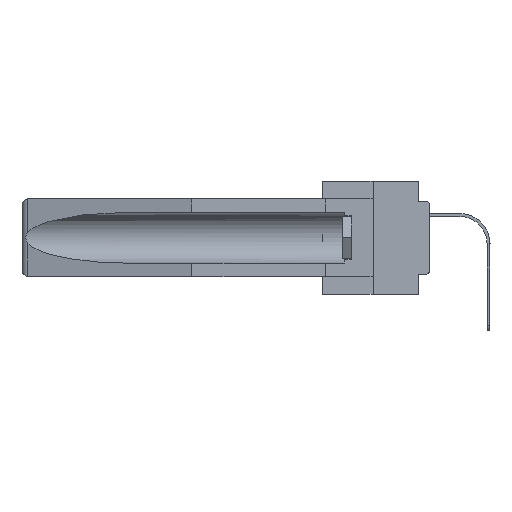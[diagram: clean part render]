
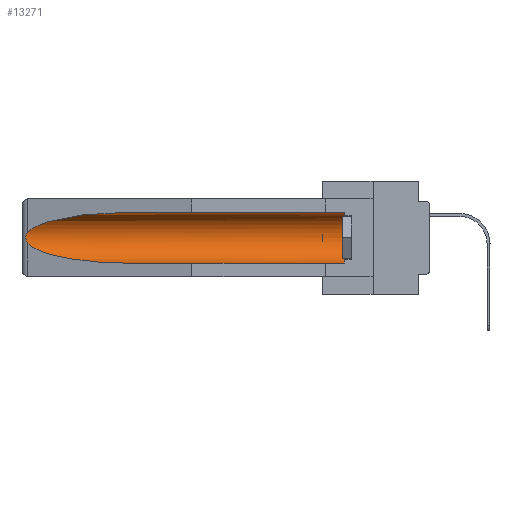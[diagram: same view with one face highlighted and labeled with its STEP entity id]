
A CAD part, left-side view. The second image highlights one B-rep face of the part: STEP entity #13271.
In plain terms, the highlighted cylindrical face has radius 2.857 mm (diameter 5.715 mm), a partial arc.
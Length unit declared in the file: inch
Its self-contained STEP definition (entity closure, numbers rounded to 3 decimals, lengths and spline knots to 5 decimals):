
#150 = CARTESIAN_POINT ( 'NONE',  ( 0.25451, 1.48313, -0.24835 ) ) ;
#886 = CARTESIAN_POINT ( 'NONE',  ( 0.155, -0.30754, -0.1715 ) ) ;
#1097 = CYLINDRICAL_SURFACE ( 'NONE', #25781, 0.1125 ) ;
#1525 =( BOUNDED_CURVE ( )  B_SPLINE_CURVE ( 3, ( #13290, #150, #25450, #12504 ),
 .UNSPECIFIED., .F., .F. ) 
 B_SPLINE_CURVE_WITH_KNOTS ( ( 4, 4 ),
 ( 0.1948, 1.5708 ),
 .UNSPECIFIED. ) 
 CURVE ( )  GEOMETRIC_REPRESENTATION_ITEM ( )  RATIONAL_B_SPLINE_CURVE ( ( 1., 0.848, 0.848, 1. ) ) 
 REPRESENTATION_ITEM ( '' )  );
#1773 = ORIENTED_EDGE ( 'NONE', *, *, #26833, .T. ) ;
#2119 = CARTESIAN_POINT ( 'NONE',  ( 0.26597, 1.5296, -0.19026 ) ) ;
#2319 = CARTESIAN_POINT ( 'NONE',  ( 0.2675, 1.53308, -0.16763 ) ) ;
#3517 = CARTESIAN_POINT ( 'NONE',  ( 0.26537, 1.52718, -0.19328 ) ) ;
#3877 = VERTEX_POINT ( 'NONE', #23800 ) ;
#5103 = DIRECTION ( 'NONE',  ( 0., 1., 0. ) ) ;
#5175 = CARTESIAN_POINT ( 'NONE',  ( 0.2673, 1.5327, -0.16383 ) ) ;
#5711 = ORIENTED_EDGE ( 'NONE', *, *, #33424, .T. ) ;
#6101 = VECTOR ( 'NONE', #5103, 39.37008 ) ;
#7322 = CARTESIAN_POINT ( 'NONE',  ( 0.155, 1.07973, -0.059 ) ) ;
#7371 = DIRECTION ( 'NONE',  ( 0., 1., 0. ) ) ;
#7547 = VERTEX_POINT ( 'NONE', #15818 ) ;
#7668 = CARTESIAN_POINT ( 'NONE',  ( 0.155, 0.126, -0.1715 ) ) ;
#8197 = CARTESIAN_POINT ( 'NONE',  ( 0.26537, 1.52718, -0.14972 ) ) ;
#8432 = DIRECTION ( 'NONE',  ( 0., 1., 0. ) ) ;
#8518 = LINE ( 'NONE', #27559, #6101 ) ;
#9685 = VERTEX_POINT ( 'NONE', #21277 ) ;
#9773 = EDGE_LOOP ( 'NONE', ( #1773, #10721, #37394, #25872, #37414, #5711 ) ) ;
#10721 = ORIENTED_EDGE ( 'NONE', *, *, #16939, .T. ) ;
#11472 = CARTESIAN_POINT ( 'NONE',  ( 0.155, -0.30754, -0.059 ) ) ;
#12179 = AXIS2_PLACEMENT_3D ( 'NONE', #7668, #26083, #20226 ) ;
#12504 = CARTESIAN_POINT ( 'NONE',  ( 0.155, 1.07973, -0.284 ) ) ;
#13271 = ADVANCED_FACE ( 'NONE', ( #28650 ), #1097, .F. ) ;
#13290 = CARTESIAN_POINT ( 'NONE',  ( 0.26537, 1.52718, -0.19328 ) ) ;
#13549 = CARTESIAN_POINT ( 'NONE',  ( 0.155, 0.126, -0.059 ) ) ;
#13828 = DIRECTION ( 'NONE',  ( 0., 0., 1. ) ) ;
#15818 = CARTESIAN_POINT ( 'NONE',  ( 0.155, 1.07973, -0.284 ) ) ;
#16831 = B_SPLINE_CURVE_WITH_KNOTS ( 'NONE', 3,
 ( #8197, #20567, #30084, #5175, #2319, #27030, #17516, #29884, #2119, #3517 ),
 .UNSPECIFIED., .F., .F.,
 ( 4, 2, 2, 2, 4 ),
 ( 0., 0.00029, 0.00058, 0.00087, 0.00117 ),
 .UNSPECIFIED. ) ;
#16939 = EDGE_CURVE ( 'NONE', #3877, #18873, #16831, .T. ) ;
#17449 = VERTEX_POINT ( 'NONE', #13549 ) ;
#17516 = CARTESIAN_POINT ( 'NONE',  ( 0.2673, 1.53269, -0.17917 ) ) ;
#17677 = EDGE_CURVE ( 'NONE', #18873, #7547, #1525, .T. ) ;
#18806 = VECTOR ( 'NONE', #8432, 39.37008 ) ;
#18873 = VERTEX_POINT ( 'NONE', #26953 ) ;
#19395 =( BOUNDED_CURVE ( )  B_SPLINE_CURVE ( 3, ( #7322, #23318, #32636, #38497 ),
 .UNSPECIFIED., .F., .F. ) 
 B_SPLINE_CURVE_WITH_KNOTS ( ( 4, 4 ),
 ( 4.71239, 6.08839 ),
 .UNSPECIFIED. ) 
 CURVE ( )  GEOMETRIC_REPRESENTATION_ITEM ( )  RATIONAL_B_SPLINE_CURVE ( ( 1., 0.848, 0.848, 1. ) ) 
 REPRESENTATION_ITEM ( '' )  );
#20226 = DIRECTION ( 'NONE',  ( 0., 0., 1. ) ) ;
#20567 = CARTESIAN_POINT ( 'NONE',  ( 0.26597, 1.52961, -0.15275 ) ) ;
#21277 = CARTESIAN_POINT ( 'NONE',  ( 0.155, 1.07973, -0.059 ) ) ;
#23318 = CARTESIAN_POINT ( 'NONE',  ( 0.21114, 1.30732, -0.059 ) ) ;
#23800 = CARTESIAN_POINT ( 'NONE',  ( 0.26537, 1.52718, -0.14972 ) ) ;
#25024 = EDGE_CURVE ( 'NONE', #29589, #17449, #29668, .T. ) ;
#25450 = CARTESIAN_POINT ( 'NONE',  ( 0.21114, 1.30732, -0.284 ) ) ;
#25781 = AXIS2_PLACEMENT_3D ( 'NONE', #886, #7371, #13828 ) ;
#25872 = ORIENTED_EDGE ( 'NONE', *, *, #38791, .F. ) ;
#26083 = DIRECTION ( 'NONE',  ( 0., -1., 0. ) ) ;
#26833 = EDGE_CURVE ( 'NONE', #9685, #3877, #19395, .T. ) ;
#26953 = CARTESIAN_POINT ( 'NONE',  ( 0.26537, 1.52718, -0.19328 ) ) ;
#27030 = CARTESIAN_POINT ( 'NONE',  ( 0.2675, 1.53308, -0.17534 ) ) ;
#27559 = CARTESIAN_POINT ( 'NONE',  ( 0.155, -0.30754, -0.284 ) ) ;
#28650 = FACE_OUTER_BOUND ( 'NONE', #9773, .T. ) ;
#29589 = VERTEX_POINT ( 'NONE', #39500 ) ;
#29668 = CIRCLE ( 'NONE', #12179, 0.1125 ) ;
#29884 = CARTESIAN_POINT ( 'NONE',  ( 0.26655, 1.53094, -0.18657 ) ) ;
#29923 = LINE ( 'NONE', #11472, #18806 ) ;
#30084 = CARTESIAN_POINT ( 'NONE',  ( 0.26654, 1.53092, -0.15636 ) ) ;
#32636 = CARTESIAN_POINT ( 'NONE',  ( 0.25451, 1.48313, -0.09465 ) ) ;
#33424 = EDGE_CURVE ( 'NONE', #17449, #9685, #29923, .T. ) ;
#37394 = ORIENTED_EDGE ( 'NONE', *, *, #17677, .T. ) ;
#37414 = ORIENTED_EDGE ( 'NONE', *, *, #25024, .T. ) ;
#38497 = CARTESIAN_POINT ( 'NONE',  ( 0.26537, 1.52718, -0.14972 ) ) ;
#38791 = EDGE_CURVE ( 'NONE', #29589, #7547, #8518, .T. ) ;
#39500 = CARTESIAN_POINT ( 'NONE',  ( 0.155, 0.126, -0.284 ) ) ;
